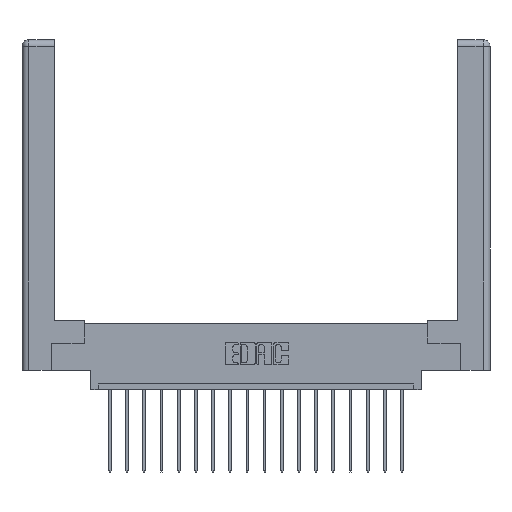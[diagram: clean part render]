
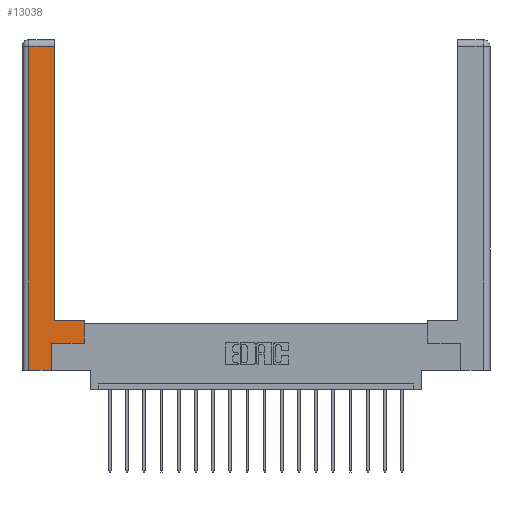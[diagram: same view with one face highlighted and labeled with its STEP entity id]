
A CAD part, top view. The second image highlights one B-rep face of the part: STEP entity #13038.
In plain terms, the highlighted planar face has unit normal (0, 0, 1).
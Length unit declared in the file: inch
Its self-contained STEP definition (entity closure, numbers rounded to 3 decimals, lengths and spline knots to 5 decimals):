
#31 = EDGE_CURVE ( 'NONE', #13573, #6723, #176, .T. ) ;
#176 = LINE ( 'NONE', #1339, #13036 ) ;
#351 = EDGE_CURVE ( 'NONE', #6723, #6852, #6933, .T. ) ;
#508 = VECTOR ( 'NONE', #11428, 39.37008 ) ;
#531 = CARTESIAN_POINT ( 'NONE',  ( 0.0615, 2.94, 0. ) ) ;
#776 = AXIS2_PLACEMENT_3D ( 'NONE', #10336, #2975, #14838 ) ;
#1339 = CARTESIAN_POINT ( 'NONE',  ( 0.265, 0., 0. ) ) ;
#1350 = ORIENTED_EDGE ( 'NONE', *, *, #16888, .T. ) ;
#1856 = CARTESIAN_POINT ( 'NONE',  ( 0.265, 0.245, 0. ) ) ;
#1875 = VECTOR ( 'NONE', #7387, 39.37008 ) ;
#2144 = CARTESIAN_POINT ( 'NONE',  ( 0.295, 2.94, 0. ) ) ;
#2378 = EDGE_CURVE ( 'NONE', #5172, #5477, #15313, .T. ) ;
#2861 = CARTESIAN_POINT ( 'NONE',  ( 0.565, 0.45, 0. ) ) ;
#2975 = DIRECTION ( 'NONE',  ( 0., 0., -1. ) ) ;
#3113 = VECTOR ( 'NONE', #13656, 39.37008 ) ;
#3391 = VERTEX_POINT ( 'NONE', #531 ) ;
#3770 = LINE ( 'NONE', #18039, #11283 ) ;
#4281 = EDGE_CURVE ( 'NONE', #14742, #3391, #3770, .T. ) ;
#4373 = CARTESIAN_POINT ( 'NONE',  ( 0.565, 0.245, 0. ) ) ;
#4450 = ORIENTED_EDGE ( 'NONE', *, *, #351, .T. ) ;
#4544 = CARTESIAN_POINT ( 'NONE',  ( 0.295, 0.45, 0. ) ) ;
#4570 = EDGE_LOOP ( 'NONE', ( #9376, #9947, #1350, #17538, #4450, #5165, #5676, #9969 ) ) ;
#4589 = CARTESIAN_POINT ( 'NONE',  ( 0.565, 0.245, 0. ) ) ;
#5165 = ORIENTED_EDGE ( 'NONE', *, *, #10303, .T. ) ;
#5172 = VERTEX_POINT ( 'NONE', #4589 ) ;
#5180 = LINE ( 'NONE', #8407, #508 ) ;
#5477 = VERTEX_POINT ( 'NONE', #2861 ) ;
#5676 = ORIENTED_EDGE ( 'NONE', *, *, #2378, .T. ) ;
#5840 = DIRECTION ( 'NONE',  ( 1., 0., 0. ) ) ;
#5855 = LINE ( 'NONE', #4373, #1875 ) ;
#6107 = DIRECTION ( 'NONE',  ( -1., 0., 0. ) ) ;
#6160 = CARTESIAN_POINT ( 'NONE',  ( 0.265, 0.245, 0. ) ) ;
#6690 = CARTESIAN_POINT ( 'NONE',  ( 0.0615, 0., 0. ) ) ;
#6723 = VERTEX_POINT ( 'NONE', #12719 ) ;
#6852 = VERTEX_POINT ( 'NONE', #6160 ) ;
#6933 = LINE ( 'NONE', #1856, #12314 ) ;
#7130 = CARTESIAN_POINT ( 'NONE',  ( 0.565, 0.45, 0. ) ) ;
#7387 = DIRECTION ( 'NONE',  ( 1., 0., 0. ) ) ;
#7698 = VERTEX_POINT ( 'NONE', #16547 ) ;
#8407 = CARTESIAN_POINT ( 'NONE',  ( 0.0615, 0., 0. ) ) ;
#9376 = ORIENTED_EDGE ( 'NONE', *, *, #10205, .T. ) ;
#9910 = LINE ( 'NONE', #4544, #3113 ) ;
#9947 = ORIENTED_EDGE ( 'NONE', *, *, #4281, .T. ) ;
#9955 = DIRECTION ( 'NONE',  ( 0., 1., 0. ) ) ;
#9969 = ORIENTED_EDGE ( 'NONE', *, *, #14140, .T. ) ;
#10205 = EDGE_CURVE ( 'NONE', #7698, #14742, #16807, .T. ) ;
#10303 = EDGE_CURVE ( 'NONE', #6852, #5172, #5855, .T. ) ;
#10336 = CARTESIAN_POINT ( 'NONE',  ( 0., 0., 0. ) ) ;
#11283 = VECTOR ( 'NONE', #6107, 39.37008 ) ;
#11335 = VECTOR ( 'NONE', #9955, 39.37008 ) ;
#11428 = DIRECTION ( 'NONE',  ( 0., -1., 0. ) ) ;
#12314 = VECTOR ( 'NONE', #13702, 39.37008 ) ;
#12719 = CARTESIAN_POINT ( 'NONE',  ( 0.265, 0., 0. ) ) ;
#13036 = VECTOR ( 'NONE', #5840, 39.37008 ) ;
#13038 = ADVANCED_FACE ( 'NONE', ( #16702 ), #17799, .F. ) ;
#13480 = DIRECTION ( 'NONE',  ( 0., 1., 0. ) ) ;
#13573 = VERTEX_POINT ( 'NONE', #6690 ) ;
#13656 = DIRECTION ( 'NONE',  ( -1., 0., 0. ) ) ;
#13702 = DIRECTION ( 'NONE',  ( 0., 1., 0. ) ) ;
#14140 = EDGE_CURVE ( 'NONE', #5477, #7698, #9910, .T. ) ;
#14742 = VERTEX_POINT ( 'NONE', #2144 ) ;
#14838 = DIRECTION ( 'NONE',  ( -1., 0., 0. ) ) ;
#15257 = VECTOR ( 'NONE', #13480, 39.37008 ) ;
#15313 = LINE ( 'NONE', #7130, #11335 ) ;
#16547 = CARTESIAN_POINT ( 'NONE',  ( 0.295, 0.45, 0. ) ) ;
#16702 = FACE_OUTER_BOUND ( 'NONE', #4570, .T. ) ;
#16807 = LINE ( 'NONE', #19285, #15257 ) ;
#16888 = EDGE_CURVE ( 'NONE', #3391, #13573, #5180, .T. ) ;
#17538 = ORIENTED_EDGE ( 'NONE', *, *, #31, .T. ) ;
#17799 = PLANE ( 'NONE',  #776 ) ;
#18039 = CARTESIAN_POINT ( 'NONE',  ( 0.0615, 2.94, 0. ) ) ;
#19285 = CARTESIAN_POINT ( 'NONE',  ( 0.295, 3., 0. ) ) ;
